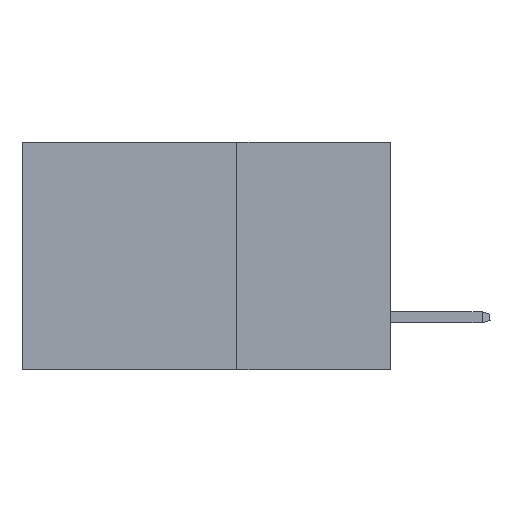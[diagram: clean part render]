
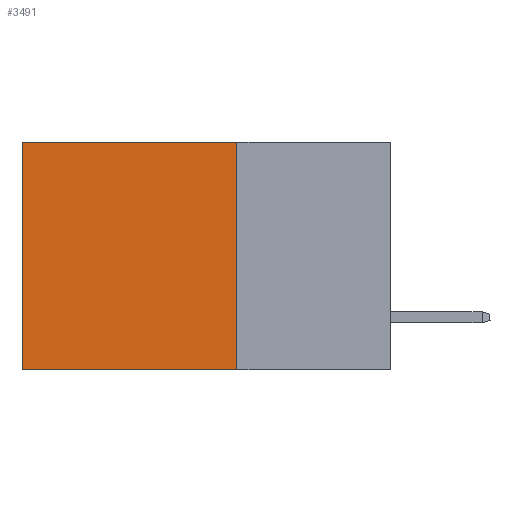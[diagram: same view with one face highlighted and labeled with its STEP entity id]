
A CAD part, left-side view. The second image highlights one B-rep face of the part: STEP entity #3491.
In plain terms, the highlighted planar face has unit normal (-1, 0, 0).
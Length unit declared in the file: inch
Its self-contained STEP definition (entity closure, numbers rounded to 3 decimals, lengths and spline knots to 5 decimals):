
#2277 = EDGE_CURVE ( 'NONE', #5584, #11979, #26273, .T. ) ;
#2606 = VERTEX_POINT ( 'NONE', #17257 ) ;
#2975 = AXIS2_PLACEMENT_3D ( 'NONE', #14783, #43533, #25657 ) ;
#3491 = ADVANCED_FACE ( 'NONE', ( #30691 ), #7462, .F. ) ;
#4066 = VECTOR ( 'NONE', #36159, 39.37008 ) ;
#5584 = VERTEX_POINT ( 'NONE', #34562 ) ;
#6851 = LINE ( 'NONE', #42183, #4066 ) ;
#7462 = PLANE ( 'NONE',  #2975 ) ;
#9568 = LINE ( 'NONE', #35114, #25857 ) ;
#10489 = DIRECTION ( 'NONE',  ( 0., 1., 0. ) ) ;
#11979 = VERTEX_POINT ( 'NONE', #45440 ) ;
#14617 = CARTESIAN_POINT ( 'NONE',  ( 0.2875, 0.6, 0. ) ) ;
#14771 = LINE ( 'NONE', #33278, #36166 ) ;
#14783 = CARTESIAN_POINT ( 'NONE',  ( 0.2875, 0.25, 0. ) ) ;
#16003 = ORIENTED_EDGE ( 'NONE', *, *, #29014, .F. ) ;
#17257 = CARTESIAN_POINT ( 'NONE',  ( 0.2875, 0.6, -0.37 ) ) ;
#18248 = DIRECTION ( 'NONE',  ( 0., 1., 0. ) ) ;
#21826 = ORIENTED_EDGE ( 'NONE', *, *, #35012, .T. ) ;
#25657 = DIRECTION ( 'NONE',  ( 0., 0., -1. ) ) ;
#25857 = VECTOR ( 'NONE', #18248, 39.37008 ) ;
#25935 = CARTESIAN_POINT ( 'NONE',  ( 0.2875, 0.25, 0. ) ) ;
#26273 = LINE ( 'NONE', #25935, #31366 ) ;
#29014 = EDGE_CURVE ( 'NONE', #11979, #2606, #14771, .T. ) ;
#30691 = FACE_OUTER_BOUND ( 'NONE', #39754, .T. ) ;
#31366 = VECTOR ( 'NONE', #40016, 39.37008 ) ;
#33278 = CARTESIAN_POINT ( 'NONE',  ( 0.2875, 0.25, -0.37 ) ) ;
#33813 = VERTEX_POINT ( 'NONE', #14617 ) ;
#34562 = CARTESIAN_POINT ( 'NONE',  ( 0.2875, 0.25, 0. ) ) ;
#35012 = EDGE_CURVE ( 'NONE', #5584, #33813, #9568, .T. ) ;
#35059 = ORIENTED_EDGE ( 'NONE', *, *, #39099, .T. ) ;
#35114 = CARTESIAN_POINT ( 'NONE',  ( 0.2875, 0.25, 0. ) ) ;
#36159 = DIRECTION ( 'NONE',  ( 0., 0., -1. ) ) ;
#36166 = VECTOR ( 'NONE', #10489, 39.37008 ) ;
#38426 = ORIENTED_EDGE ( 'NONE', *, *, #2277, .F. ) ;
#39099 = EDGE_CURVE ( 'NONE', #33813, #2606, #6851, .T. ) ;
#39754 = EDGE_LOOP ( 'NONE', ( #35059, #16003, #38426, #21826 ) ) ;
#40016 = DIRECTION ( 'NONE',  ( 0., 0., -1. ) ) ;
#42183 = CARTESIAN_POINT ( 'NONE',  ( 0.2875, 0.6, 0. ) ) ;
#43533 = DIRECTION ( 'NONE',  ( 1., 0., 0. ) ) ;
#45440 = CARTESIAN_POINT ( 'NONE',  ( 0.2875, 0.25, -0.37 ) ) ;
